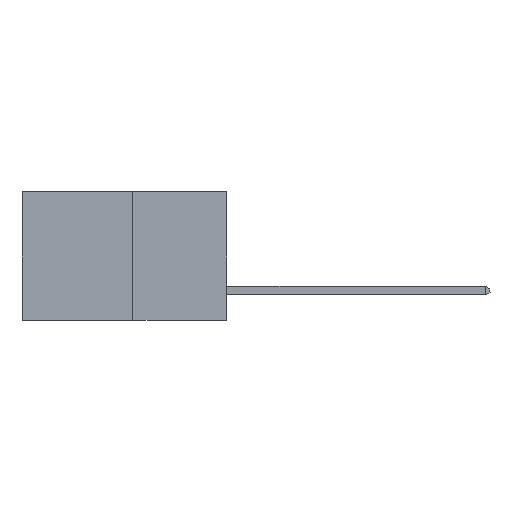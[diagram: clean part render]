
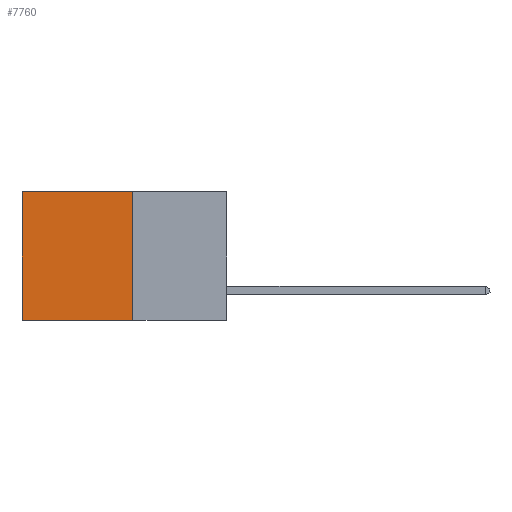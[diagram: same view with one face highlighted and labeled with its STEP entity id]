
A CAD part, left-side view. The second image highlights one B-rep face of the part: STEP entity #7760.
In plain terms, the highlighted planar face has unit normal (-1, 0, 0).
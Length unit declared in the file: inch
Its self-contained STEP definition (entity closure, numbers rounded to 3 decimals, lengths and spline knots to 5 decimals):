
#503 = VERTEX_POINT ( 'NONE', #1901 ) ;
#712 = EDGE_CURVE ( 'NONE', #4375, #9700, #6074, .T. ) ;
#971 = EDGE_CURVE ( 'NONE', #9700, #8851, #11432, .T. ) ;
#1122 = CARTESIAN_POINT ( 'NONE',  ( 0.277, 0.27, -0.37 ) ) ;
#1388 = ORIENTED_EDGE ( 'NONE', *, *, #5300, .T. ) ;
#1901 = CARTESIAN_POINT ( 'NONE',  ( 0.277, 0.59, 0. ) ) ;
#2448 = VECTOR ( 'NONE', #6902, 39.37008 ) ;
#2560 = EDGE_LOOP ( 'NONE', ( #1388, #10494, #5542, #13033 ) ) ;
#4375 = VERTEX_POINT ( 'NONE', #11361 ) ;
#4598 = PLANE ( 'NONE',  #6172 ) ;
#4989 = DIRECTION ( 'NONE',  ( 0., 1., 0. ) ) ;
#5300 = EDGE_CURVE ( 'NONE', #503, #8851, #10745, .T. ) ;
#5424 = EDGE_CURVE ( 'NONE', #4375, #503, #6025, .T. ) ;
#5542 = ORIENTED_EDGE ( 'NONE', *, *, #712, .F. ) ;
#6025 = LINE ( 'NONE', #8264, #11137 ) ;
#6074 = LINE ( 'NONE', #1122, #8273 ) ;
#6172 = AXIS2_PLACEMENT_3D ( 'NONE', #12355, #6855, #13186 ) ;
#6855 = DIRECTION ( 'NONE',  ( 1., 0., 0. ) ) ;
#6902 = DIRECTION ( 'NONE',  ( 0., 0., -1. ) ) ;
#7395 = DIRECTION ( 'NONE',  ( 0., 0., -1. ) ) ;
#7760 = ADVANCED_FACE ( 'NONE', ( #7771 ), #4598, .F. ) ;
#7771 = FACE_OUTER_BOUND ( 'NONE', #2560, .T. ) ;
#8264 = CARTESIAN_POINT ( 'NONE',  ( 0.277, 0.27, 0. ) ) ;
#8273 = VECTOR ( 'NONE', #7395, 39.37008 ) ;
#8510 = CARTESIAN_POINT ( 'NONE',  ( 0.277, 0.27, -0.37 ) ) ;
#8851 = VERTEX_POINT ( 'NONE', #10197 ) ;
#9700 = VERTEX_POINT ( 'NONE', #10888 ) ;
#10197 = CARTESIAN_POINT ( 'NONE',  ( 0.277, 0.59, -0.37 ) ) ;
#10494 = ORIENTED_EDGE ( 'NONE', *, *, #971, .F. ) ;
#10745 = LINE ( 'NONE', #11538, #2448 ) ;
#10888 = CARTESIAN_POINT ( 'NONE',  ( 0.277, 0.27, -0.37 ) ) ;
#11137 = VECTOR ( 'NONE', #4989, 39.37008 ) ;
#11167 = VECTOR ( 'NONE', #12250, 39.37008 ) ;
#11361 = CARTESIAN_POINT ( 'NONE',  ( 0.277, 0.27, 0. ) ) ;
#11432 = LINE ( 'NONE', #8510, #11167 ) ;
#11538 = CARTESIAN_POINT ( 'NONE',  ( 0.277, 0.59, -0.37 ) ) ;
#12250 = DIRECTION ( 'NONE',  ( 0., 1., 0. ) ) ;
#12355 = CARTESIAN_POINT ( 'NONE',  ( 0.277, 0.27, -0.37 ) ) ;
#13033 = ORIENTED_EDGE ( 'NONE', *, *, #5424, .T. ) ;
#13186 = DIRECTION ( 'NONE',  ( 0., 0., -1. ) ) ;
